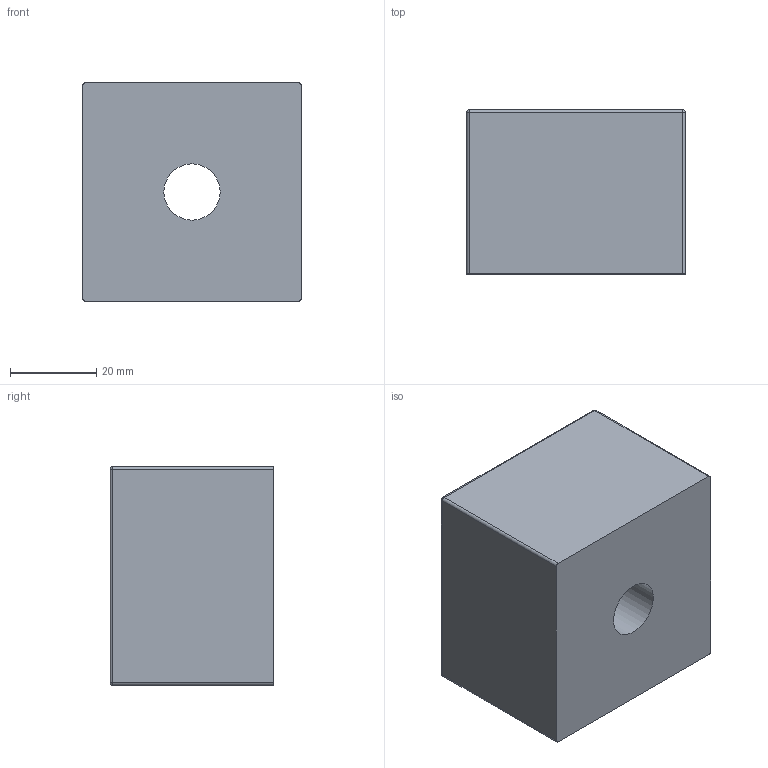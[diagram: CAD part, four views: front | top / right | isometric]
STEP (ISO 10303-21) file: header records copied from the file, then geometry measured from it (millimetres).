
FILE_DESCRIPTION(/* description */ (''),/* implementation_level */ '2;1');
FILE_NAME(/* name */ 'Jig 2.stp',/* time_stamp */ '2019-03-23T15:16:17-05:00',/* author */ ('johne'),/* organization */ (''),/* preprocessor_version */ 'ST-DEVELOPER v16.13',/* originating_system */ 'Autodesk Inventor 2018',/* authorisation */ '');
FILE_SCHEMA (('AUTOMOTIVE_DESIGN { 1 0 10303 214 3 1 1 }'));
Length unit declared in the file: inch
Products named in the file (1): Jig 2
Bounding box: 50.8 x 38.1 x 50.8 mm (x, y, z)
Volume: 84948.5 mm3; surface area: 15269 mm2
Topology: 1 solids, 1 shells, 62 faces, 150 edges, 92 vertices
Faces by surface type: plane 22, cylinder 21, bspline 11, sphere 4, torus 4
Full cylindrical faces by diameter (mm): 13.081 x1
Entity records: 1966 total; most frequent: CARTESIAN_POINT 547, ORIENTED_EDGE 298, DIRECTION 257, EDGE_CURVE 149, VERTEX_POINT 92, AXIS2_PLACEMENT_3D 86, LINE 85, VECTOR 85
